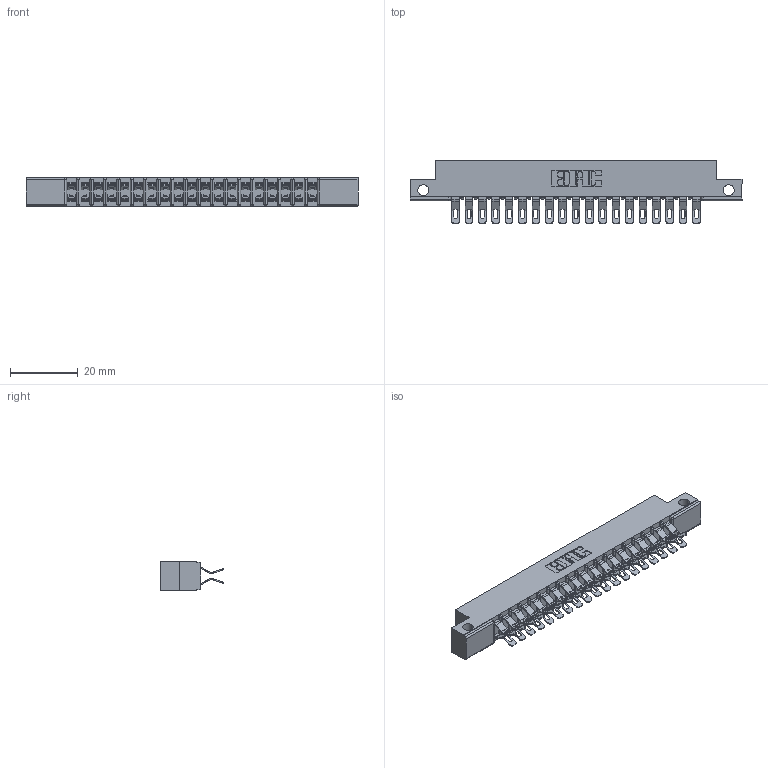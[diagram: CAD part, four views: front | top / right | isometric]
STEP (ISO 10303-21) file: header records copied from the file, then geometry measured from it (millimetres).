
FILE_DESCRIPTION (( 'STEP AP203' ), '1' );
FILE_NAME ('307-038-555-212.STEP', '2019-09-06T04:41:34', ( '' ), ( '' ), 'SwSTEP 2.0', 'SolidWorks 2016', '' );
FILE_SCHEMA (( 'CONFIG_CONTROL_DESIGN' ));
Length unit declared in the file: inch
Products named in the file (3): 307-290-001_555; 307 Part_.128 Dia Side Mounting Holes; 307-038-555-212
Assembly tree (39 placements, depth 2):
  307-038-555-212
    307 Part_.128 Dia Side Mounting Holes
    307-290-001_555  x38
Bounding box: 98.3 x 18.75 x 8.71 mm (x, y, z)
Volume: 6467.4 mm3; surface area: 11753.6 mm2
Topology: 39 solids, 39 shells, 2456 faces, 7201 edges, 4694 vertices
Faces by surface type: plane 1362, cylinder 1054, sphere 40
Entity records: 20271 total; most frequent: CARTESIAN_POINT 3327, ORIENTED_EDGE 3296, DIRECTION 3276, EDGE_CURVE 1648, VECTOR 1242, LINE 1242, VERTEX_POINT 1068, AXIS2_PLACEMENT_3D 1017
